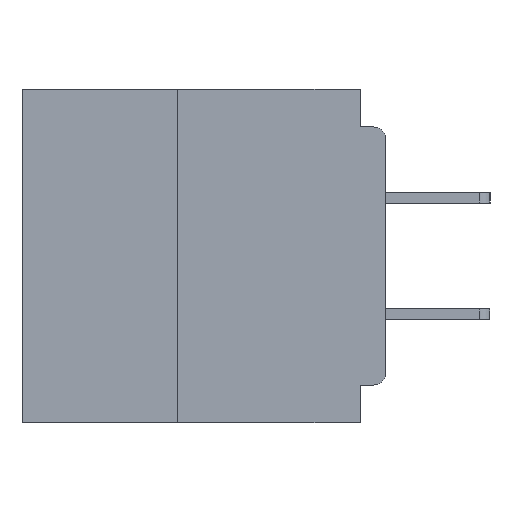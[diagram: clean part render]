
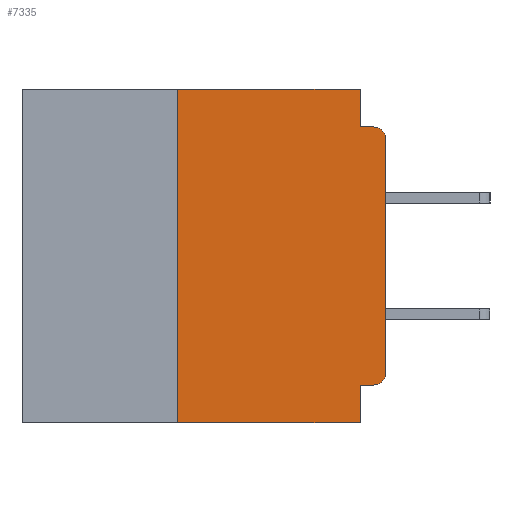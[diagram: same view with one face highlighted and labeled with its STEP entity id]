
A CAD part, left-side view. The second image highlights one B-rep face of the part: STEP entity #7335.
In plain terms, the highlighted planar face has unit normal (-1, 0, 0).
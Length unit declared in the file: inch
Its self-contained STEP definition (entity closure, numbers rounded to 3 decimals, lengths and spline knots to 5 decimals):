
#84 = VECTOR ( 'NONE', #15205, 39.37008 ) ;
#164 = VERTEX_POINT ( 'NONE', #19080 ) ;
#343 = DIRECTION ( 'NONE',  ( 0., -1., 0. ) ) ;
#349 = CIRCLE ( 'NONE', #10448, 0.015 ) ;
#471 = LINE ( 'NONE', #20748, #15848 ) ;
#627 = VECTOR ( 'NONE', #24226, 39.37008 ) ;
#1365 = ORIENTED_EDGE ( 'NONE', *, *, #24856, .T. ) ;
#1673 = CARTESIAN_POINT ( 'NONE',  ( 0., 0., 0. ) ) ;
#2058 = LINE ( 'NONE', #33399, #84 ) ;
#2487 = CARTESIAN_POINT ( 'NONE',  ( 0., 0., -0.355 ) ) ;
#2856 = ORIENTED_EDGE ( 'NONE', *, *, #12922, .T. ) ;
#3074 = DIRECTION ( 'NONE',  ( -1., 0., 0. ) ) ;
#3913 = VERTEX_POINT ( 'NONE', #32436 ) ;
#4002 = LINE ( 'NONE', #21789, #12154 ) ;
#4776 = VECTOR ( 'NONE', #32086, 39.37008 ) ;
#5018 = LINE ( 'NONE', #1673, #35450 ) ;
#5481 = DIRECTION ( 'NONE',  ( 0., -1., 0. ) ) ;
#5568 = VERTEX_POINT ( 'NONE', #17502 ) ;
#5954 = CARTESIAN_POINT ( 'NONE',  ( 0., 0.031, -0.045 ) ) ;
#6214 = ORIENTED_EDGE ( 'NONE', *, *, #30538, .F. ) ;
#7335 = ADVANCED_FACE ( 'NONE', ( #37239 ), #21533, .F. ) ;
#7381 = CARTESIAN_POINT ( 'NONE',  ( 0., 0.031, 0. ) ) ;
#7769 = CARTESIAN_POINT ( 'NONE',  ( 0., 0.015, -0.06 ) ) ;
#7895 = EDGE_CURVE ( 'NONE', #164, #5568, #2058, .T. ) ;
#9102 = ORIENTED_EDGE ( 'NONE', *, *, #29777, .F. ) ;
#10068 = LINE ( 'NONE', #2487, #26277 ) ;
#10448 = AXIS2_PLACEMENT_3D ( 'NONE', #7769, #29099, #10856 ) ;
#10856 = DIRECTION ( 'NONE',  ( 0., 0., -1. ) ) ;
#12154 = VECTOR ( 'NONE', #343, 39.37008 ) ;
#12569 = CARTESIAN_POINT ( 'NONE',  ( 0., 0.031, 0. ) ) ;
#12572 = VECTOR ( 'NONE', #36778, 39.37008 ) ;
#12922 = EDGE_CURVE ( 'NONE', #14768, #5568, #30082, .T. ) ;
#13244 = EDGE_LOOP ( 'NONE', ( #1365, #18670, #35647, #6214, #32410, #9102, #2856, #35200, #36138, #14848 ) ) ;
#14436 = CARTESIAN_POINT ( 'NONE',  ( 0., 0.015, -0.355 ) ) ;
#14768 = VERTEX_POINT ( 'NONE', #37951 ) ;
#14848 = ORIENTED_EDGE ( 'NONE', *, *, #15070, .T. ) ;
#15070 = EDGE_CURVE ( 'NONE', #34976, #25733, #26353, .T. ) ;
#15205 = DIRECTION ( 'NONE',  ( 0., 0., -1. ) ) ;
#15525 = CARTESIAN_POINT ( 'NONE',  ( 0., 0.437, 0. ) ) ;
#15848 = VECTOR ( 'NONE', #5481, 39.37008 ) ;
#16035 = AXIS2_PLACEMENT_3D ( 'NONE', #15525, #36650, #18608 ) ;
#16972 = LINE ( 'NONE', #27285, #627 ) ;
#17502 = CARTESIAN_POINT ( 'NONE',  ( 0., 0.031, -0.4 ) ) ;
#18608 = DIRECTION ( 'NONE',  ( 0., 0., -1. ) ) ;
#18670 = ORIENTED_EDGE ( 'NONE', *, *, #27398, .T. ) ;
#19080 = CARTESIAN_POINT ( 'NONE',  ( 0., 0.031, -0.355 ) ) ;
#19133 = EDGE_CURVE ( 'NONE', #39216, #25930, #4002, .T. ) ;
#19911 = CARTESIAN_POINT ( 'NONE',  ( 0., 0.437, -0.4 ) ) ;
#20724 = LINE ( 'NONE', #12569, #12572 ) ;
#20748 = CARTESIAN_POINT ( 'NONE',  ( 0., 0., -0.045 ) ) ;
#21315 = EDGE_CURVE ( 'NONE', #34976, #164, #10068, .T. ) ;
#21418 = CARTESIAN_POINT ( 'NONE',  ( 0., 0.015, -0.34 ) ) ;
#21533 = PLANE ( 'NONE',  #16035 ) ;
#21789 = CARTESIAN_POINT ( 'NONE',  ( 0., 0.437, 0. ) ) ;
#22423 = CARTESIAN_POINT ( 'NONE',  ( 0., 0.015, -0.045 ) ) ;
#23265 = CARTESIAN_POINT ( 'NONE',  ( 0., 0.25, 0. ) ) ;
#23861 = DIRECTION ( 'NONE',  ( 0., 1., 0. ) ) ;
#24226 = DIRECTION ( 'NONE',  ( 0., 0., 1. ) ) ;
#24455 = DIRECTION ( 'NONE',  ( 0., 0., -1. ) ) ;
#24856 = EDGE_CURVE ( 'NONE', #25733, #3913, #5018, .T. ) ;
#25733 = VERTEX_POINT ( 'NONE', #39051 ) ;
#25930 = VERTEX_POINT ( 'NONE', #7381 ) ;
#26131 = EDGE_CURVE ( 'NONE', #28352, #37270, #471, .T. ) ;
#26139 = DIRECTION ( 'NONE',  ( 0., 0., 1. ) ) ;
#26277 = VECTOR ( 'NONE', #23861, 39.37008 ) ;
#26353 = CIRCLE ( 'NONE', #34901, 0.015 ) ;
#27285 = CARTESIAN_POINT ( 'NONE',  ( 0., 0.25, -0.4 ) ) ;
#27398 = EDGE_CURVE ( 'NONE', #3913, #37270, #349, .T. ) ;
#28352 = VERTEX_POINT ( 'NONE', #5954 ) ;
#29099 = DIRECTION ( 'NONE',  ( -1., 0., 0. ) ) ;
#29777 = EDGE_CURVE ( 'NONE', #14768, #39216, #16972, .T. ) ;
#30082 = LINE ( 'NONE', #19911, #4776 ) ;
#30538 = EDGE_CURVE ( 'NONE', #25930, #28352, #20724, .T. ) ;
#32086 = DIRECTION ( 'NONE',  ( 0., -1., 0. ) ) ;
#32410 = ORIENTED_EDGE ( 'NONE', *, *, #19133, .F. ) ;
#32436 = CARTESIAN_POINT ( 'NONE',  ( 0., 0., -0.06 ) ) ;
#33399 = CARTESIAN_POINT ( 'NONE',  ( 0., 0.031, -0.4 ) ) ;
#34901 = AXIS2_PLACEMENT_3D ( 'NONE', #21418, #3074, #24455 ) ;
#34976 = VERTEX_POINT ( 'NONE', #14436 ) ;
#35200 = ORIENTED_EDGE ( 'NONE', *, *, #7895, .F. ) ;
#35450 = VECTOR ( 'NONE', #26139, 39.37008 ) ;
#35647 = ORIENTED_EDGE ( 'NONE', *, *, #26131, .F. ) ;
#36138 = ORIENTED_EDGE ( 'NONE', *, *, #21315, .F. ) ;
#36650 = DIRECTION ( 'NONE',  ( 1., 0., 0. ) ) ;
#36778 = DIRECTION ( 'NONE',  ( 0., 0., -1. ) ) ;
#37239 = FACE_OUTER_BOUND ( 'NONE', #13244, .T. ) ;
#37270 = VERTEX_POINT ( 'NONE', #22423 ) ;
#37951 = CARTESIAN_POINT ( 'NONE',  ( 0., 0.25, -0.4 ) ) ;
#39051 = CARTESIAN_POINT ( 'NONE',  ( 0., 0., -0.34 ) ) ;
#39216 = VERTEX_POINT ( 'NONE', #23265 ) ;
